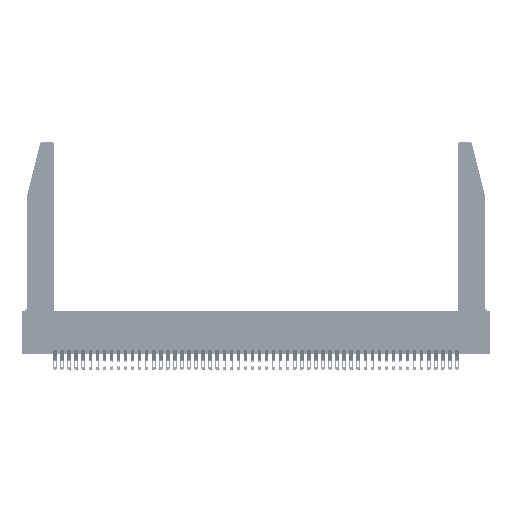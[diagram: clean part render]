
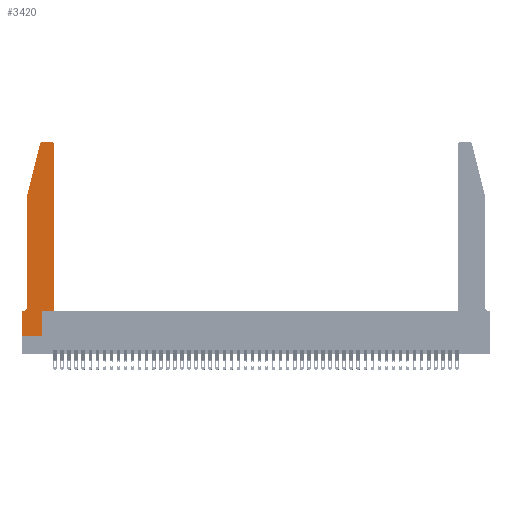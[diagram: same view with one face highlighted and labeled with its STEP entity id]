
A CAD part, top view. The second image highlights one B-rep face of the part: STEP entity #3420.
In plain terms, the highlighted planar face has unit normal (0, 0, 1).
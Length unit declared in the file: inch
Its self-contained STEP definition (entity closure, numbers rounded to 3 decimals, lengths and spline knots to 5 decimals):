
#219 = DIRECTION ( 'NONE',  ( -1., 0., 0. ) ) ;
#736 = CARTESIAN_POINT ( 'NONE',  ( 0.2605, 2.75, 0.37 ) ) ;
#1303 = VECTOR ( 'NONE', #45913, 39.37008 ) ;
#1859 = LINE ( 'NONE', #34996, #41069 ) ;
#2076 = EDGE_CURVE ( 'NONE', #40511, #27943, #47423, .T. ) ;
#2131 = VERTEX_POINT ( 'NONE', #12840 ) ;
#2166 = EDGE_CURVE ( 'NONE', #27943, #42443, #11275, .T. ) ;
#2564 = DIRECTION ( 'NONE',  ( -1., 0., 0. ) ) ;
#2595 = EDGE_CURVE ( 'NONE', #34517, #3281, #33182, .T. ) ;
#2856 = DIRECTION ( 'NONE',  ( 1., 0., 0. ) ) ;
#2909 = CARTESIAN_POINT ( 'NONE',  ( 0.4505, 2.72, 0.37 ) ) ;
#2939 = CARTESIAN_POINT ( 'NONE',  ( 0., 0., 0.37 ) ) ;
#3281 = VERTEX_POINT ( 'NONE', #4429 ) ;
#3420 = ADVANCED_FACE ( 'NONE', ( #6188 ), #35413, .T. ) ;
#3705 = CARTESIAN_POINT ( 'NONE',  ( 0.4505, 0.35, 0.37 ) ) ;
#4218 = EDGE_LOOP ( 'NONE', ( #19738, #8633, #43561, #20855, #46919, #39291, #6202, #42274, #43594, #5851, #40377, #14147 ) ) ;
#4429 = CARTESIAN_POINT ( 'NONE',  ( 0., 0., 0.37 ) ) ;
#5456 = VECTOR ( 'NONE', #7127, 39.37008 ) ;
#5581 = CIRCLE ( 'NONE', #9828, 0.03 ) ;
#5851 = ORIENTED_EDGE ( 'NONE', *, *, #6019, .T. ) ;
#6019 = EDGE_CURVE ( 'NONE', #10823, #23909, #11202, .T. ) ;
#6188 = FACE_OUTER_BOUND ( 'NONE', #4218, .T. ) ;
#6202 = ORIENTED_EDGE ( 'NONE', *, *, #2595, .T. ) ;
#7127 = DIRECTION ( 'NONE',  ( -1., 0., 0. ) ) ;
#7351 = CARTESIAN_POINT ( 'NONE',  ( 0.0055, 0.35, 0.37 ) ) ;
#8138 = CARTESIAN_POINT ( 'NONE',  ( 0.2865, 0.35, 0.37 ) ) ;
#8633 = ORIENTED_EDGE ( 'NONE', *, *, #41784, .T. ) ;
#8765 = CARTESIAN_POINT ( 'NONE',  ( 0.4505, 0.35, 0.37 ) ) ;
#9057 = AXIS2_PLACEMENT_3D ( 'NONE', #32271, #10047, #2856 ) ;
#9566 = CARTESIAN_POINT ( 'NONE',  ( 0.2865, 0., 0.37 ) ) ;
#9828 = AXIS2_PLACEMENT_3D ( 'NONE', #40449, #10984, #40909 ) ;
#10047 = DIRECTION ( 'NONE',  ( 0., 0., 1. ) ) ;
#10073 = VERTEX_POINT ( 'NONE', #22598 ) ;
#10667 = AXIS2_PLACEMENT_3D ( 'NONE', #36521, #28811, #29290 ) ;
#10823 = VERTEX_POINT ( 'NONE', #8138 ) ;
#10984 = DIRECTION ( 'NONE',  ( 0., 0., 1. ) ) ;
#11202 = LINE ( 'NONE', #37891, #1303 ) ;
#11275 = CIRCLE ( 'NONE', #36283, 0.07 ) ;
#12840 = CARTESIAN_POINT ( 'NONE',  ( 0.4205, 2.75, 0.37 ) ) ;
#13049 = LINE ( 'NONE', #736, #13663 ) ;
#13311 = CARTESIAN_POINT ( 'NONE',  ( 0.0055, 0.42, 0.37 ) ) ;
#13512 = EDGE_CURVE ( 'NONE', #28690, #10823, #1859, .T. ) ;
#13663 = VECTOR ( 'NONE', #219, 39.37008 ) ;
#13805 = DIRECTION ( 'NONE',  ( 0., 1., 0. ) ) ;
#14147 = ORIENTED_EDGE ( 'NONE', *, *, #22483, .T. ) ;
#16447 = DIRECTION ( 'NONE',  ( 0., -1., 0. ) ) ;
#17547 = VECTOR ( 'NONE', #16447, 39.37008 ) ;
#17809 = VECTOR ( 'NONE', #33854, 39.37008 ) ;
#17958 = CARTESIAN_POINT ( 'NONE',  ( 0.0755, 2., 0.37 ) ) ;
#18980 = LINE ( 'NONE', #40552, #17809 ) ;
#19738 = ORIENTED_EDGE ( 'NONE', *, *, #38532, .T. ) ;
#20756 = CARTESIAN_POINT ( 'NONE',  ( 0.0755, 0.42, 0.37 ) ) ;
#20855 = ORIENTED_EDGE ( 'NONE', *, *, #2076, .T. ) ;
#22483 = EDGE_CURVE ( 'NONE', #47405, #2131, #48028, .T. ) ;
#22598 = CARTESIAN_POINT ( 'NONE',  ( 0.284, 2.75, 0.37 ) ) ;
#23909 = VERTEX_POINT ( 'NONE', #8765 ) ;
#26080 = CARTESIAN_POINT ( 'NONE',  ( 0.0755, 0.35, 0.37 ) ) ;
#26377 = LINE ( 'NONE', #41475, #46293 ) ;
#27567 = CARTESIAN_POINT ( 'NONE',  ( 0., 0.35, 0.37 ) ) ;
#27943 = VERTEX_POINT ( 'NONE', #20756 ) ;
#28075 = DIRECTION ( 'NONE',  ( 0., 1., 0. ) ) ;
#28569 = DIRECTION ( 'NONE',  ( 0., -1., 0. ) ) ;
#28690 = VERTEX_POINT ( 'NONE', #9566 ) ;
#28811 = DIRECTION ( 'NONE',  ( 0., 0., 1. ) ) ;
#29290 = DIRECTION ( 'NONE',  ( 1., 0., 0. ) ) ;
#29621 = VECTOR ( 'NONE', #28569, 39.37008 ) ;
#32234 = VERTEX_POINT ( 'NONE', #48175 ) ;
#32271 = CARTESIAN_POINT ( 'NONE',  ( 0., 0.35, 0.37 ) ) ;
#33182 = LINE ( 'NONE', #2939, #29621 ) ;
#33854 = DIRECTION ( 'NONE',  ( 1., 0., 0. ) ) ;
#34517 = VERTEX_POINT ( 'NONE', #27567 ) ;
#34996 = CARTESIAN_POINT ( 'NONE',  ( 0.2865, 0.35, 0.37 ) ) ;
#35106 = CARTESIAN_POINT ( 'NONE',  ( 0.0755, 2., 0.37 ) ) ;
#35413 = PLANE ( 'NONE',  #9057 ) ;
#36283 = AXIS2_PLACEMENT_3D ( 'NONE', #13311, #47665, #2564 ) ;
#36521 = CARTESIAN_POINT ( 'NONE',  ( 0.4205, 2.72, 0.37 ) ) ;
#37071 = DIRECTION ( 'NONE',  ( -0.239, -0.971, 0. ) ) ;
#37078 = VECTOR ( 'NONE', #13805, 39.37008 ) ;
#37891 = CARTESIAN_POINT ( 'NONE',  ( 0.4505, 0.35, 0.37 ) ) ;
#38457 = EDGE_CURVE ( 'NONE', #23909, #47405, #42352, .T. ) ;
#38532 = EDGE_CURVE ( 'NONE', #2131, #10073, #13049, .T. ) ;
#39291 = ORIENTED_EDGE ( 'NONE', *, *, #43967, .T. ) ;
#39826 = EDGE_CURVE ( 'NONE', #32234, #40511, #26377, .T. ) ;
#40377 = ORIENTED_EDGE ( 'NONE', *, *, #38457, .T. ) ;
#40449 = CARTESIAN_POINT ( 'NONE',  ( 0.284, 2.72, 0.37 ) ) ;
#40511 = VERTEX_POINT ( 'NONE', #17958 ) ;
#40538 = LINE ( 'NONE', #26080, #5456 ) ;
#40552 = CARTESIAN_POINT ( 'NONE',  ( 0., 0., 0.37 ) ) ;
#40909 = DIRECTION ( 'NONE',  ( 1., 0., 0. ) ) ;
#41069 = VECTOR ( 'NONE', #28075, 39.37008 ) ;
#41475 = CARTESIAN_POINT ( 'NONE',  ( 0.0755, 2., 0.37 ) ) ;
#41784 = EDGE_CURVE ( 'NONE', #10073, #32234, #5581, .T. ) ;
#42274 = ORIENTED_EDGE ( 'NONE', *, *, #42416, .T. ) ;
#42352 = LINE ( 'NONE', #3705, #37078 ) ;
#42416 = EDGE_CURVE ( 'NONE', #3281, #28690, #18980, .T. ) ;
#42443 = VERTEX_POINT ( 'NONE', #7351 ) ;
#43561 = ORIENTED_EDGE ( 'NONE', *, *, #39826, .T. ) ;
#43594 = ORIENTED_EDGE ( 'NONE', *, *, #13512, .T. ) ;
#43967 = EDGE_CURVE ( 'NONE', #42443, #34517, #40538, .T. ) ;
#45913 = DIRECTION ( 'NONE',  ( 1., 0., 0. ) ) ;
#46293 = VECTOR ( 'NONE', #37071, 39.37008 ) ;
#46919 = ORIENTED_EDGE ( 'NONE', *, *, #2166, .T. ) ;
#47405 = VERTEX_POINT ( 'NONE', #2909 ) ;
#47423 = LINE ( 'NONE', #35106, #17547 ) ;
#47665 = DIRECTION ( 'NONE',  ( 0., 0., -1. ) ) ;
#48028 = CIRCLE ( 'NONE', #10667, 0.03 ) ;
#48175 = CARTESIAN_POINT ( 'NONE',  ( 0.25487, 2.72718, 0.37 ) ) ;
